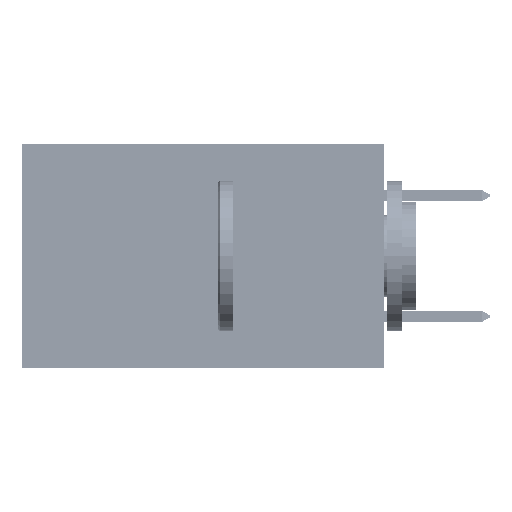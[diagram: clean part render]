
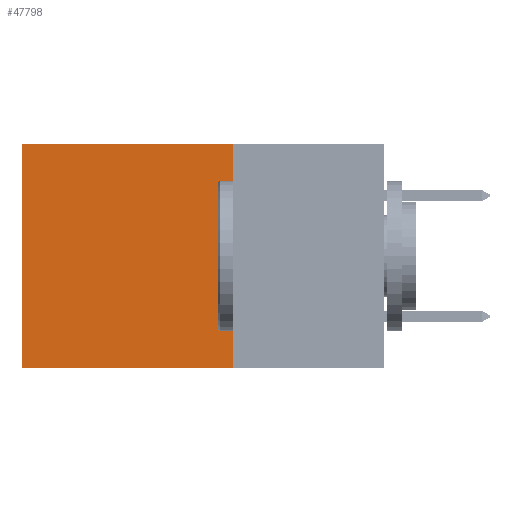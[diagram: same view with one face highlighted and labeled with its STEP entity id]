
A CAD part, left-side view. The second image highlights one B-rep face of the part: STEP entity #47798.
In plain terms, the highlighted planar face has unit normal (-1, 0, 0).
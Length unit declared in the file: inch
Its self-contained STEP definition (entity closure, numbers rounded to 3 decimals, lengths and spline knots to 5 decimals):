
#274 = PLANE ( 'NONE',  #8422 ) ;
#1482 = FACE_OUTER_BOUND ( 'NONE', #27579, .T. ) ;
#2068 = VERTEX_POINT ( 'NONE', #25186 ) ;
#2602 = DIRECTION ( 'NONE',  ( 0., 1., 0. ) ) ;
#2710 = DIRECTION ( 'NONE',  ( 0., 0., -1. ) ) ;
#4167 = DIRECTION ( 'NONE',  ( 1., 0., 0. ) ) ;
#5622 = DIRECTION ( 'NONE',  ( 0., 0., -1. ) ) ;
#6755 = CARTESIAN_POINT ( 'NONE',  ( 0.2875, 0.25, 0. ) ) ;
#7221 = CARTESIAN_POINT ( 'NONE',  ( 0.2875, 0.25, 0. ) ) ;
#7933 = CARTESIAN_POINT ( 'NONE',  ( 0.2875, 0.25, 0. ) ) ;
#8422 = AXIS2_PLACEMENT_3D ( 'NONE', #7933, #4167, #31545 ) ;
#9566 = EDGE_CURVE ( 'NONE', #10329, #2068, #12304, .T. ) ;
#10329 = VERTEX_POINT ( 'NONE', #7221 ) ;
#12304 = LINE ( 'NONE', #6755, #43494 ) ;
#14156 = EDGE_CURVE ( 'NONE', #19167, #20138, #14939, .T. ) ;
#14939 = LINE ( 'NONE', #26042, #44885 ) ;
#19167 = VERTEX_POINT ( 'NONE', #36915 ) ;
#20096 = ORIENTED_EDGE ( 'NONE', *, *, #14156, .F. ) ;
#20138 = VERTEX_POINT ( 'NONE', #50536 ) ;
#20417 = VECTOR ( 'NONE', #5622, 39.37008 ) ;
#21050 = EDGE_CURVE ( 'NONE', #2068, #20138, #29588, .T. ) ;
#23403 = CARTESIAN_POINT ( 'NONE',  ( 0.2875, 0.25, 0. ) ) ;
#25186 = CARTESIAN_POINT ( 'NONE',  ( 0.2875, 0.6, 0. ) ) ;
#26042 = CARTESIAN_POINT ( 'NONE',  ( 0.2875, 0.25, -0.37 ) ) ;
#27579 = EDGE_LOOP ( 'NONE', ( #34650, #20096, #32290, #36897 ) ) ;
#29080 = CARTESIAN_POINT ( 'NONE',  ( 0.2875, 0.6, 0. ) ) ;
#29588 = LINE ( 'NONE', #29080, #20417 ) ;
#31545 = DIRECTION ( 'NONE',  ( 0., 0., -1. ) ) ;
#32290 = ORIENTED_EDGE ( 'NONE', *, *, #47045, .F. ) ;
#34129 = DIRECTION ( 'NONE',  ( 0., 1., 0. ) ) ;
#34650 = ORIENTED_EDGE ( 'NONE', *, *, #21050, .T. ) ;
#36897 = ORIENTED_EDGE ( 'NONE', *, *, #9566, .T. ) ;
#36915 = CARTESIAN_POINT ( 'NONE',  ( 0.2875, 0.25, -0.37 ) ) ;
#40325 = VECTOR ( 'NONE', #2710, 39.37008 ) ;
#43494 = VECTOR ( 'NONE', #34129, 39.37008 ) ;
#44885 = VECTOR ( 'NONE', #2602, 39.37008 ) ;
#47045 = EDGE_CURVE ( 'NONE', #10329, #19167, #49527, .T. ) ;
#47798 = ADVANCED_FACE ( 'NONE', ( #1482 ), #274, .F. ) ;
#49527 = LINE ( 'NONE', #23403, #40325 ) ;
#50536 = CARTESIAN_POINT ( 'NONE',  ( 0.2875, 0.6, -0.37 ) ) ;
